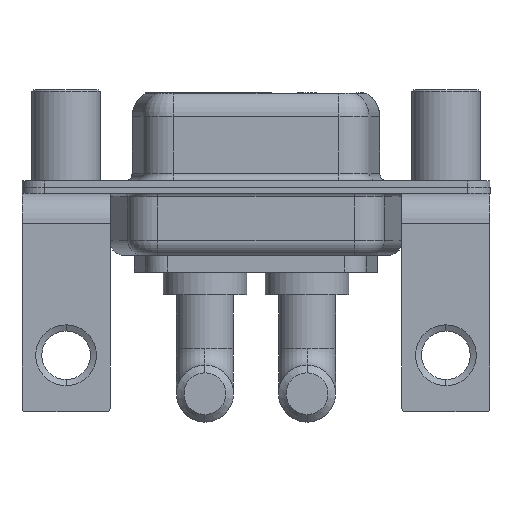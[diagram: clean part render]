
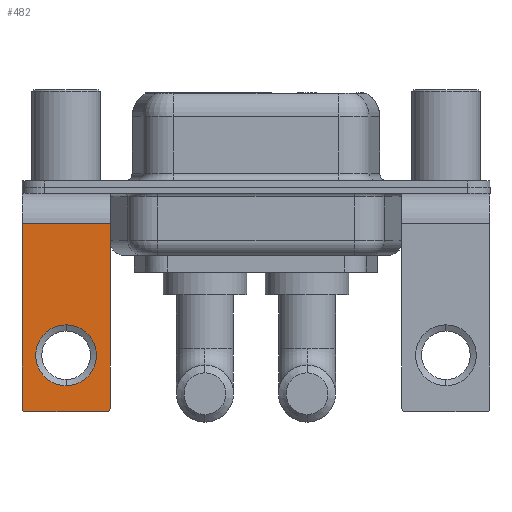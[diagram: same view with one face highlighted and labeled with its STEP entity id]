
A CAD part, front view. The second image highlights one B-rep face of the part: STEP entity #482.
In plain terms, the highlighted planar face has unit normal (0, -1, 0).
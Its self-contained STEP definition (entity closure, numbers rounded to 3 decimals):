
#482 = ADVANCED_FACE ( 'NONE', ( #9011, #13887 ), #7813, .F. ) ;
#499 = CARTESIAN_POINT ( 'NONE',  ( 0., -6.25, -13.07 ) ) ;
#623 = AXIS2_PLACEMENT_3D ( 'NONE', #8051, #3070, #11666 ) ;
#646 = CARTESIAN_POINT ( 'NONE',  ( 0., -6.25, -9.07 ) ) ;
#683 = EDGE_CURVE ( 'NONE', #950, #10593, #7453, .T. ) ;
#734 = VERTEX_POINT ( 'NONE', #8524 ) ;
#908 = VECTOR ( 'NONE', #12876, 1000. ) ;
#945 = LINE ( 'NONE', #8001, #908 ) ;
#950 = VERTEX_POINT ( 'NONE', #499 ) ;
#1480 = DIRECTION ( 'NONE',  ( 0., -1., 0. ) ) ;
#1562 = AXIS2_PLACEMENT_3D ( 'NONE', #10789, #9328, #15637 ) ;
#1699 = CARTESIAN_POINT ( 'NONE',  ( -2.9, -6.25, -14.55 ) ) ;
#2173 = AXIS2_PLACEMENT_3D ( 'NONE', #6370, #1480, #11267 ) ;
#2443 = VERTEX_POINT ( 'NONE', #14534 ) ;
#2782 = ORIENTED_EDGE ( 'NONE', *, *, #6018, .T. ) ;
#2829 = CARTESIAN_POINT ( 'NONE',  ( 2.9, -6.25, -2.4 ) ) ;
#2839 = CARTESIAN_POINT ( 'NONE',  ( -2.9, -6.25, -2.4 ) ) ;
#3070 = DIRECTION ( 'NONE',  ( 0., 1., 0. ) ) ;
#3205 = ORIENTED_EDGE ( 'NONE', *, *, #13061, .F. ) ;
#3419 = CARTESIAN_POINT ( 'NONE',  ( 2.9, -6.25, -2.4 ) ) ;
#3535 = VERTEX_POINT ( 'NONE', #11723 ) ;
#4178 = LINE ( 'NONE', #2829, #12411 ) ;
#4382 = EDGE_CURVE ( 'NONE', #8089, #8008, #13809, .T. ) ;
#4496 = DIRECTION ( 'NONE',  ( 0., 0., 1. ) ) ;
#4699 = CARTESIAN_POINT ( 'NONE',  ( 2.9, -6.25, -2.4 ) ) ;
#5282 = EDGE_LOOP ( 'NONE', ( #12138, #10804, #3205, #9840, #5576, #15591 ) ) ;
#5576 = ORIENTED_EDGE ( 'NONE', *, *, #14406, .F. ) ;
#5799 = VECTOR ( 'NONE', #9595, 1000. ) ;
#5800 = EDGE_CURVE ( 'NONE', #734, #3535, #12655, .T. ) ;
#5846 = ORIENTED_EDGE ( 'NONE', *, *, #683, .T. ) ;
#6018 = EDGE_CURVE ( 'NONE', #10593, #950, #10096, .T. ) ;
#6355 = AXIS2_PLACEMENT_3D ( 'NONE', #12988, #13222, #4496 ) ;
#6370 = CARTESIAN_POINT ( 'NONE',  ( 2.65, -6.25, -14.55 ) ) ;
#6599 = DIRECTION ( 'NONE',  ( -1., 0., 0. ) ) ;
#7325 = CARTESIAN_POINT ( 'NONE',  ( 0., -6.25, -11.07 ) ) ;
#7453 = CIRCLE ( 'NONE', #10005, 2. ) ;
#7731 = DIRECTION ( 'NONE',  ( 0., 0., -1. ) ) ;
#7813 = PLANE ( 'NONE',  #1562 ) ;
#8001 = CARTESIAN_POINT ( 'NONE',  ( 2.9, -6.25, -14.8 ) ) ;
#8008 = VERTEX_POINT ( 'NONE', #1699 ) ;
#8051 = CARTESIAN_POINT ( 'NONE',  ( 0., -6.25, -11.07 ) ) ;
#8089 = VERTEX_POINT ( 'NONE', #13077 ) ;
#8524 = CARTESIAN_POINT ( 'NONE',  ( 2.65, -6.25, -14.8 ) ) ;
#8554 = LINE ( 'NONE', #4699, #5799 ) ;
#9011 = FACE_BOUND ( 'NONE', #10257, .T. ) ;
#9328 = DIRECTION ( 'NONE',  ( 0., 1., 0. ) ) ;
#9595 = DIRECTION ( 'NONE',  ( 0., 0., -1. ) ) ;
#9840 = ORIENTED_EDGE ( 'NONE', *, *, #5800, .T. ) ;
#10005 = AXIS2_PLACEMENT_3D ( 'NONE', #7325, #12199, #11017 ) ;
#10096 = CIRCLE ( 'NONE', #623, 2. ) ;
#10180 = EDGE_CURVE ( 'NONE', #11606, #8089, #4178, .T. ) ;
#10257 = EDGE_LOOP ( 'NONE', ( #5846, #2782 ) ) ;
#10593 = VERTEX_POINT ( 'NONE', #646 ) ;
#10789 = CARTESIAN_POINT ( 'NONE',  ( 2.9, -6.25, -2.4 ) ) ;
#10804 = ORIENTED_EDGE ( 'NONE', *, *, #10839, .T. ) ;
#10839 = EDGE_CURVE ( 'NONE', #8008, #2443, #13262, .T. ) ;
#11017 = DIRECTION ( 'NONE',  ( 0., 0., 1. ) ) ;
#11267 = DIRECTION ( 'NONE',  ( 0., 0., 1. ) ) ;
#11606 = VERTEX_POINT ( 'NONE', #3419 ) ;
#11666 = DIRECTION ( 'NONE',  ( 0., 0., 1. ) ) ;
#11723 = CARTESIAN_POINT ( 'NONE',  ( 2.9, -6.25, -14.55 ) ) ;
#12138 = ORIENTED_EDGE ( 'NONE', *, *, #4382, .T. ) ;
#12199 = DIRECTION ( 'NONE',  ( 0., 1., 0. ) ) ;
#12411 = VECTOR ( 'NONE', #6599, 1000. ) ;
#12655 = CIRCLE ( 'NONE', #2173, 0.25 ) ;
#12876 = DIRECTION ( 'NONE',  ( -1., 0., 0. ) ) ;
#12988 = CARTESIAN_POINT ( 'NONE',  ( -2.65, -6.25, -14.55 ) ) ;
#13061 = EDGE_CURVE ( 'NONE', #734, #2443, #945, .T. ) ;
#13077 = CARTESIAN_POINT ( 'NONE',  ( -2.9, -6.25, -2.4 ) ) ;
#13222 = DIRECTION ( 'NONE',  ( 0., -1., 0. ) ) ;
#13262 = CIRCLE ( 'NONE', #6355, 0.25 ) ;
#13809 = LINE ( 'NONE', #2839, #14403 ) ;
#13887 = FACE_OUTER_BOUND ( 'NONE', #5282, .T. ) ;
#14403 = VECTOR ( 'NONE', #7731, 1000. ) ;
#14406 = EDGE_CURVE ( 'NONE', #11606, #3535, #8554, .T. ) ;
#14534 = CARTESIAN_POINT ( 'NONE',  ( -2.65, -6.25, -14.8 ) ) ;
#15591 = ORIENTED_EDGE ( 'NONE', *, *, #10180, .T. ) ;
#15637 = DIRECTION ( 'NONE',  ( 0., 0., 1. ) ) ;
